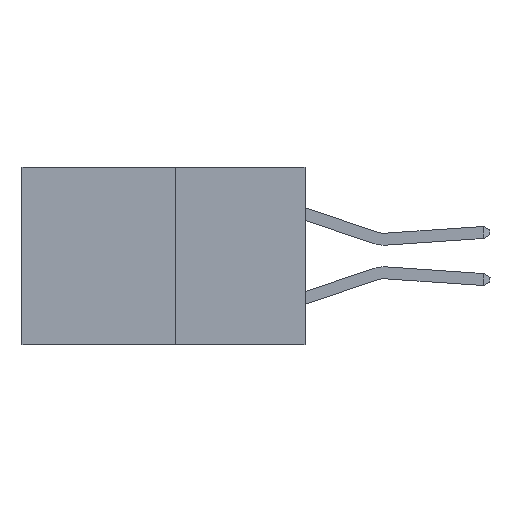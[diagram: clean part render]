
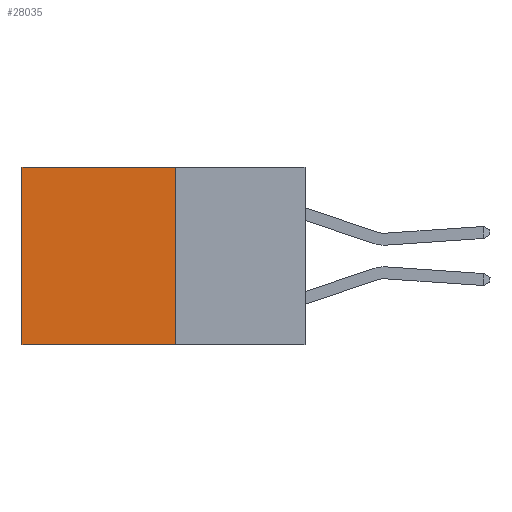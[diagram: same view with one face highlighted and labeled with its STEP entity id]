
A CAD part, left-side view. The second image highlights one B-rep face of the part: STEP entity #28035.
In plain terms, the highlighted planar face has unit normal (-1, 0, 0).
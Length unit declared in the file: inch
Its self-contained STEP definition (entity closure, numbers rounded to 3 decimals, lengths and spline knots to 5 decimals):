
#881 = DIRECTION ( 'NONE',  ( 1., 0., 0. ) ) ;
#992 = CARTESIAN_POINT ( 'NONE',  ( 0.277, 0.59, -0.37 ) ) ;
#1462 = CARTESIAN_POINT ( 'NONE',  ( 0.277, 0.27, -0.37 ) ) ;
#2123 = VERTEX_POINT ( 'NONE', #14942 ) ;
#3639 = VECTOR ( 'NONE', #5892, 39.37008 ) ;
#4449 = LINE ( 'NONE', #7216, #15433 ) ;
#4545 = VECTOR ( 'NONE', #14156, 39.37008 ) ;
#5292 = VECTOR ( 'NONE', #6526, 39.37008 ) ;
#5892 = DIRECTION ( 'NONE',  ( 0., 1., 0. ) ) ;
#6526 = DIRECTION ( 'NONE',  ( 0., 1., 0. ) ) ;
#6624 = EDGE_CURVE ( 'NONE', #2123, #26646, #4449, .T. ) ;
#7216 = CARTESIAN_POINT ( 'NONE',  ( 0.277, 0.27, -0.37 ) ) ;
#8433 = EDGE_CURVE ( 'NONE', #26646, #23491, #16005, .T. ) ;
#9095 = CARTESIAN_POINT ( 'NONE',  ( 0.277, 0.59, 0. ) ) ;
#10114 = VERTEX_POINT ( 'NONE', #9095 ) ;
#10884 = CARTESIAN_POINT ( 'NONE',  ( 0.277, 0.27, 0. ) ) ;
#12283 = DIRECTION ( 'NONE',  ( 0., 0., -1. ) ) ;
#14044 = CARTESIAN_POINT ( 'NONE',  ( 0.277, 0.27, -0.37 ) ) ;
#14156 = DIRECTION ( 'NONE',  ( 0., 0., -1. ) ) ;
#14453 = CARTESIAN_POINT ( 'NONE',  ( 0.277, 0.27, -0.37 ) ) ;
#14942 = CARTESIAN_POINT ( 'NONE',  ( 0.277, 0.27, 0. ) ) ;
#15418 = CARTESIAN_POINT ( 'NONE',  ( 0.277, 0.59, -0.37 ) ) ;
#15433 = VECTOR ( 'NONE', #12283, 39.37008 ) ;
#15531 = LINE ( 'NONE', #992, #4545 ) ;
#15711 = AXIS2_PLACEMENT_3D ( 'NONE', #14044, #881, #16251 ) ;
#16005 = LINE ( 'NONE', #1462, #3639 ) ;
#16251 = DIRECTION ( 'NONE',  ( 0., 0., -1. ) ) ;
#17158 = ORIENTED_EDGE ( 'NONE', *, *, #27031, .T. ) ;
#17323 = ORIENTED_EDGE ( 'NONE', *, *, #6624, .F. ) ;
#21729 = FACE_OUTER_BOUND ( 'NONE', #25446, .T. ) ;
#21737 = EDGE_CURVE ( 'NONE', #10114, #23491, #15531, .T. ) ;
#21764 = ORIENTED_EDGE ( 'NONE', *, *, #21737, .T. ) ;
#22676 = PLANE ( 'NONE',  #15711 ) ;
#23491 = VERTEX_POINT ( 'NONE', #15418 ) ;
#24714 = LINE ( 'NONE', #10884, #5292 ) ;
#25446 = EDGE_LOOP ( 'NONE', ( #21764, #28100, #17323, #17158 ) ) ;
#26646 = VERTEX_POINT ( 'NONE', #14453 ) ;
#27031 = EDGE_CURVE ( 'NONE', #2123, #10114, #24714, .T. ) ;
#28035 = ADVANCED_FACE ( 'NONE', ( #21729 ), #22676, .F. ) ;
#28100 = ORIENTED_EDGE ( 'NONE', *, *, #8433, .F. ) ;
